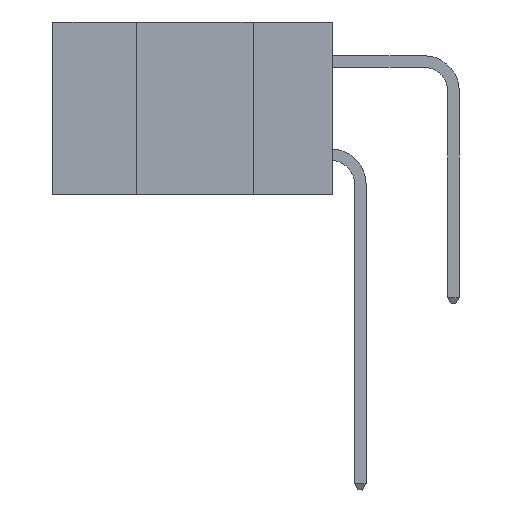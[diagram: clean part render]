
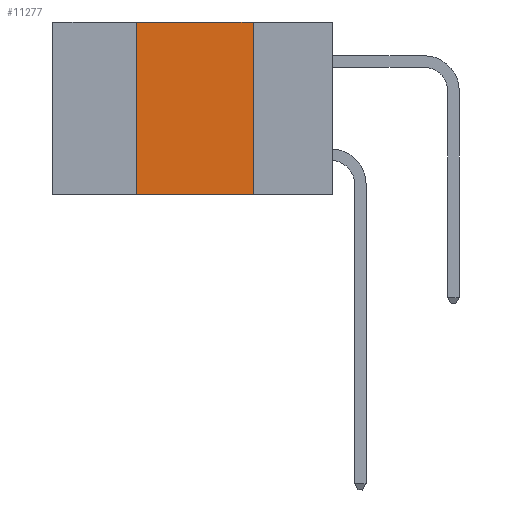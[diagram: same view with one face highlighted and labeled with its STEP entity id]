
A CAD part, left-side view. The second image highlights one B-rep face of the part: STEP entity #11277.
In plain terms, the highlighted planar face has unit normal (-1, 0, 0).
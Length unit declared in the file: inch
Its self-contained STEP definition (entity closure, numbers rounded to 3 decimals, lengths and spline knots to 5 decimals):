
#66 = CARTESIAN_POINT ( 'NONE',  ( 0., 0.17, -0.37 ) ) ;
#800 = CARTESIAN_POINT ( 'NONE',  ( 0., 0.6, 0. ) ) ;
#1322 = EDGE_CURVE ( 'NONE', #1574, #3088, #5229, .T. ) ;
#1574 = VERTEX_POINT ( 'NONE', #9566 ) ;
#1648 = LINE ( 'NONE', #12029, #15573 ) ;
#2255 = DIRECTION ( 'NONE',  ( 0., 0., -1. ) ) ;
#2567 = ORIENTED_EDGE ( 'NONE', *, *, #1322, .T. ) ;
#2911 = DIRECTION ( 'NONE',  ( 0., 0., 1. ) ) ;
#3088 = VERTEX_POINT ( 'NONE', #66 ) ;
#4632 = EDGE_CURVE ( 'NONE', #14663, #3088, #10182, .T. ) ;
#5229 = LINE ( 'NONE', #10852, #15475 ) ;
#5358 = ORIENTED_EDGE ( 'NONE', *, *, #4632, .F. ) ;
#6653 = AXIS2_PLACEMENT_3D ( 'NONE', #800, #10314, #2255 ) ;
#6908 = EDGE_LOOP ( 'NONE', ( #5358, #12433, #16442, #2567 ) ) ;
#7098 = CARTESIAN_POINT ( 'NONE',  ( 0., 0.42, 0. ) ) ;
#8957 = PLANE ( 'NONE',  #6653 ) ;
#9566 = CARTESIAN_POINT ( 'NONE',  ( 0., 0.42, -0.37 ) ) ;
#9595 = CARTESIAN_POINT ( 'NONE',  ( 0., 0.42, 0. ) ) ;
#9745 = VECTOR ( 'NONE', #10824, 39.37008 ) ;
#10182 = LINE ( 'NONE', #11200, #9745 ) ;
#10314 = DIRECTION ( 'NONE',  ( 1., 0., 0. ) ) ;
#10637 = VECTOR ( 'NONE', #2911, 39.37008 ) ;
#10824 = DIRECTION ( 'NONE',  ( 0., 0., -1. ) ) ;
#10852 = CARTESIAN_POINT ( 'NONE',  ( 0., 0.6, -0.37 ) ) ;
#11022 = VERTEX_POINT ( 'NONE', #7098 ) ;
#11200 = CARTESIAN_POINT ( 'NONE',  ( 0., 0.17, 0. ) ) ;
#11277 = ADVANCED_FACE ( 'NONE', ( #14187 ), #8957, .F. ) ;
#12029 = CARTESIAN_POINT ( 'NONE',  ( 0., 0.6, 0. ) ) ;
#12433 = ORIENTED_EDGE ( 'NONE', *, *, #13641, .F. ) ;
#12699 = DIRECTION ( 'NONE',  ( 0., -1., 0. ) ) ;
#13641 = EDGE_CURVE ( 'NONE', #11022, #14663, #1648, .T. ) ;
#14187 = FACE_OUTER_BOUND ( 'NONE', #6908, .T. ) ;
#14617 = LINE ( 'NONE', #9595, #10637 ) ;
#14663 = VERTEX_POINT ( 'NONE', #16847 ) ;
#14813 = EDGE_CURVE ( 'NONE', #1574, #11022, #14617, .T. ) ;
#15475 = VECTOR ( 'NONE', #12699, 39.37008 ) ;
#15573 = VECTOR ( 'NONE', #16100, 39.37008 ) ;
#16100 = DIRECTION ( 'NONE',  ( 0., -1., 0. ) ) ;
#16442 = ORIENTED_EDGE ( 'NONE', *, *, #14813, .F. ) ;
#16847 = CARTESIAN_POINT ( 'NONE',  ( 0., 0.17, 0. ) ) ;
